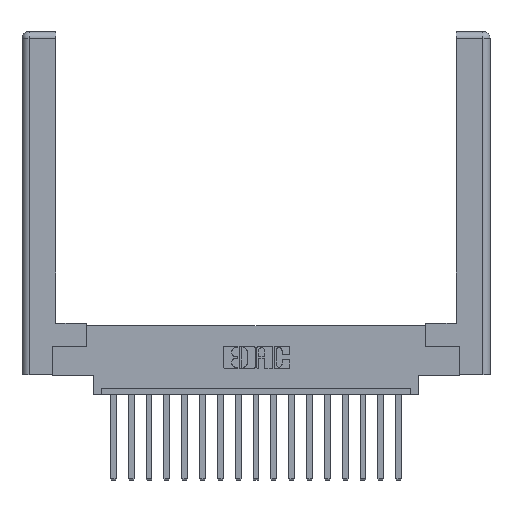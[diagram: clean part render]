
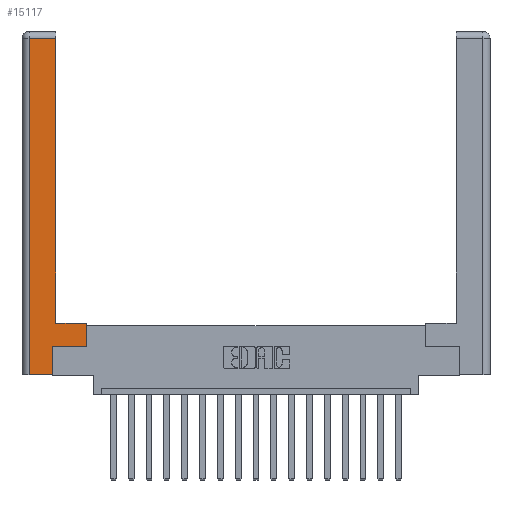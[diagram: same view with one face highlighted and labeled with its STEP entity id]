
A CAD part, top view. The second image highlights one B-rep face of the part: STEP entity #15117.
In plain terms, the highlighted planar face has unit normal (0, 0, 1).
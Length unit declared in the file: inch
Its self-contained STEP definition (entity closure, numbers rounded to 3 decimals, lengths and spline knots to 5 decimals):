
#282 = DIRECTION ( 'NONE',  ( 0., 0., -1. ) ) ;
#943 = VECTOR ( 'NONE', #2734, 39.37008 ) ;
#995 = DIRECTION ( 'NONE',  ( 1., 0., 0. ) ) ;
#1183 = VERTEX_POINT ( 'NONE', #17113 ) ;
#1210 = VECTOR ( 'NONE', #7792, 39.37008 ) ;
#1493 = VERTEX_POINT ( 'NONE', #16964 ) ;
#1520 = VERTEX_POINT ( 'NONE', #1587 ) ;
#1587 = CARTESIAN_POINT ( 'NONE',  ( 0.265, 0.245, 0. ) ) ;
#1773 = VERTEX_POINT ( 'NONE', #15773 ) ;
#1903 = PLANE ( 'NONE',  #12465 ) ;
#2547 = VECTOR ( 'NONE', #4153, 39.37008 ) ;
#2734 = DIRECTION ( 'NONE',  ( 0., 1., 0. ) ) ;
#2878 = CARTESIAN_POINT ( 'NONE',  ( 0.565, 0.245, 0. ) ) ;
#3031 = ORIENTED_EDGE ( 'NONE', *, *, #16379, .T. ) ;
#3310 = EDGE_CURVE ( 'NONE', #7855, #1183, #10353, .T. ) ;
#4149 = EDGE_CURVE ( 'NONE', #1183, #4592, #4235, .T. ) ;
#4153 = DIRECTION ( 'NONE',  ( 0., 1., 0. ) ) ;
#4219 = CARTESIAN_POINT ( 'NONE',  ( 0.565, 0.45, 0. ) ) ;
#4235 = LINE ( 'NONE', #5813, #12763 ) ;
#4592 = VERTEX_POINT ( 'NONE', #4839 ) ;
#4839 = CARTESIAN_POINT ( 'NONE',  ( 0.0615, 0., 0. ) ) ;
#5338 = VECTOR ( 'NONE', #9944, 39.37008 ) ;
#5605 = ORIENTED_EDGE ( 'NONE', *, *, #9630, .T. ) ;
#5618 = VECTOR ( 'NONE', #6942, 39.37008 ) ;
#5813 = CARTESIAN_POINT ( 'NONE',  ( 0.0615, 0., 0. ) ) ;
#6942 = DIRECTION ( 'NONE',  ( -1., 0., 0. ) ) ;
#7101 = CARTESIAN_POINT ( 'NONE',  ( 0.295, 3., 0. ) ) ;
#7107 = CARTESIAN_POINT ( 'NONE',  ( 0.295, 0.45, 0. ) ) ;
#7541 = EDGE_CURVE ( 'NONE', #1773, #7855, #17903, .T. ) ;
#7792 = DIRECTION ( 'NONE',  ( 0., 1., 0. ) ) ;
#7855 = VERTEX_POINT ( 'NONE', #9046 ) ;
#8195 = VECTOR ( 'NONE', #16653, 39.37008 ) ;
#8460 = EDGE_CURVE ( 'NONE', #1520, #17869, #15297, .T. ) ;
#8619 = ORIENTED_EDGE ( 'NONE', *, *, #3310, .T. ) ;
#9046 = CARTESIAN_POINT ( 'NONE',  ( 0.295, 2.94, 0. ) ) ;
#9596 = CARTESIAN_POINT ( 'NONE',  ( 0.265, 0., 0. ) ) ;
#9630 = EDGE_CURVE ( 'NONE', #17869, #12535, #12191, .T. ) ;
#9944 = DIRECTION ( 'NONE',  ( -1., 0., 0. ) ) ;
#10294 = CARTESIAN_POINT ( 'NONE',  ( 0.565, 0.45, 0. ) ) ;
#10353 = LINE ( 'NONE', #18255, #5618 ) ;
#11545 = EDGE_LOOP ( 'NONE', ( #11890, #8619, #12904, #12042, #3031, #18403, #5605, #12262 ) ) ;
#11556 = VECTOR ( 'NONE', #995, 39.37008 ) ;
#11890 = ORIENTED_EDGE ( 'NONE', *, *, #7541, .T. ) ;
#12042 = ORIENTED_EDGE ( 'NONE', *, *, #15883, .T. ) ;
#12191 = LINE ( 'NONE', #4219, #2547 ) ;
#12262 = ORIENTED_EDGE ( 'NONE', *, *, #13113, .T. ) ;
#12465 = AXIS2_PLACEMENT_3D ( 'NONE', #17533, #282, #14659 ) ;
#12535 = VERTEX_POINT ( 'NONE', #10294 ) ;
#12763 = VECTOR ( 'NONE', #14493, 39.37008 ) ;
#12904 = ORIENTED_EDGE ( 'NONE', *, *, #4149, .T. ) ;
#13113 = EDGE_CURVE ( 'NONE', #12535, #1773, #14736, .T. ) ;
#13826 = FACE_OUTER_BOUND ( 'NONE', #11545, .T. ) ;
#14433 = LINE ( 'NONE', #9596, #11556 ) ;
#14493 = DIRECTION ( 'NONE',  ( 0., -1., 0. ) ) ;
#14659 = DIRECTION ( 'NONE',  ( -1., 0., 0. ) ) ;
#14736 = LINE ( 'NONE', #7107, #5338 ) ;
#15117 = ADVANCED_FACE ( 'NONE', ( #13826 ), #1903, .F. ) ;
#15297 = LINE ( 'NONE', #18028, #8195 ) ;
#15773 = CARTESIAN_POINT ( 'NONE',  ( 0.295, 0.45, 0. ) ) ;
#15883 = EDGE_CURVE ( 'NONE', #4592, #1493, #14433, .T. ) ;
#16379 = EDGE_CURVE ( 'NONE', #1493, #1520, #16591, .T. ) ;
#16591 = LINE ( 'NONE', #17664, #1210 ) ;
#16653 = DIRECTION ( 'NONE',  ( 1., 0., 0. ) ) ;
#16964 = CARTESIAN_POINT ( 'NONE',  ( 0.265, 0., 0. ) ) ;
#17113 = CARTESIAN_POINT ( 'NONE',  ( 0.0615, 2.94, 0. ) ) ;
#17533 = CARTESIAN_POINT ( 'NONE',  ( 0., 0., 0. ) ) ;
#17664 = CARTESIAN_POINT ( 'NONE',  ( 0.265, 0.245, 0. ) ) ;
#17869 = VERTEX_POINT ( 'NONE', #2878 ) ;
#17903 = LINE ( 'NONE', #7101, #943 ) ;
#18028 = CARTESIAN_POINT ( 'NONE',  ( 0.565, 0.245, 0. ) ) ;
#18255 = CARTESIAN_POINT ( 'NONE',  ( 0.0615, 2.94, 0. ) ) ;
#18403 = ORIENTED_EDGE ( 'NONE', *, *, #8460, .T. ) ;
